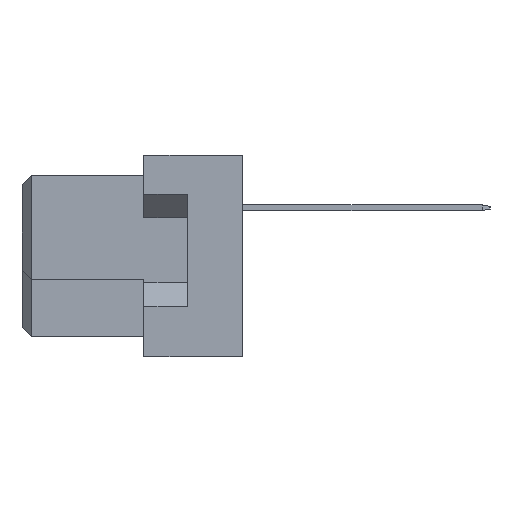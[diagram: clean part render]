
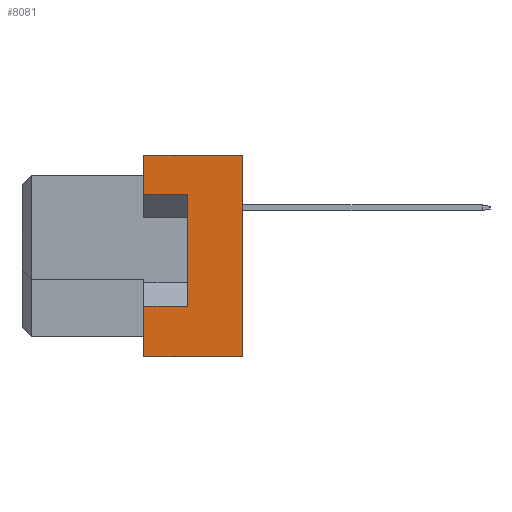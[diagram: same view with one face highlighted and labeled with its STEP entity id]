
A CAD part, left-side view. The second image highlights one B-rep face of the part: STEP entity #8081.
In plain terms, the highlighted planar face has unit normal (-1, 0, 0).
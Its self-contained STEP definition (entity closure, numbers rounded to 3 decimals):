
#211 = DIRECTION ( 'NONE',  ( 0., 0., 1. ) ) ;
#1290 = ORIENTED_EDGE ( 'NONE', *, *, #20643, .F. ) ;
#2016 = ORIENTED_EDGE ( 'NONE', *, *, #21092, .T. ) ;
#3316 = VERTEX_POINT ( 'NONE', #11749 ) ;
#4869 = CARTESIAN_POINT ( 'NONE',  ( -47.5, -11.6, 5.3 ) ) ;
#5547 = LINE ( 'NONE', #26498, #6067 ) ;
#5551 = VERTEX_POINT ( 'NONE', #25028 ) ;
#5770 = VERTEX_POINT ( 'NONE', #14816 ) ;
#5952 = DIRECTION ( 'NONE',  ( 0., 1., 0. ) ) ;
#6067 = VECTOR ( 'NONE', #8678, 1000. ) ;
#6468 = EDGE_CURVE ( 'NONE', #32099, #27374, #15330, .T. ) ;
#7495 = CARTESIAN_POINT ( 'NONE',  ( -47.5, -6.4, -2.65 ) ) ;
#7597 = DIRECTION ( 'NONE',  ( 0., 0., 1. ) ) ;
#7832 = VECTOR ( 'NONE', #8297, 1000. ) ;
#7844 = ORIENTED_EDGE ( 'NONE', *, *, #29473, .F. ) ;
#8081 = ADVANCED_FACE ( 'NONE', ( #37391 ), #34633, .T. ) ;
#8297 = DIRECTION ( 'NONE',  ( 0., 1., 0. ) ) ;
#8309 = VECTOR ( 'NONE', #35183, 1000. ) ;
#8678 = DIRECTION ( 'NONE',  ( 0., 0., 1. ) ) ;
#9259 = CARTESIAN_POINT ( 'NONE',  ( -47.5, -8.7, -2.65 ) ) ;
#11006 = VERTEX_POINT ( 'NONE', #27903 ) ;
#11712 = ORIENTED_EDGE ( 'NONE', *, *, #31493, .F. ) ;
#11749 = CARTESIAN_POINT ( 'NONE',  ( -47.5, -6.4, -5.3 ) ) ;
#12090 = VERTEX_POINT ( 'NONE', #22367 ) ;
#12371 = CARTESIAN_POINT ( 'NONE',  ( -47.5, -11.6, 5.3 ) ) ;
#12782 = VECTOR ( 'NONE', #36684, 1000. ) ;
#13508 = CARTESIAN_POINT ( 'NONE',  ( -47.5, -6.4, -5.3 ) ) ;
#14209 = CARTESIAN_POINT ( 'NONE',  ( -47.5, -11.6, -5.3 ) ) ;
#14816 = CARTESIAN_POINT ( 'NONE',  ( -47.5, -11.6, -5.3 ) ) ;
#14832 = LINE ( 'NONE', #23255, #8309 ) ;
#15099 = LINE ( 'NONE', #12371, #36594 ) ;
#15330 = LINE ( 'NONE', #27853, #12782 ) ;
#17097 = ORIENTED_EDGE ( 'NONE', *, *, #6468, .T. ) ;
#17341 = CARTESIAN_POINT ( 'NONE',  ( -47.5, -8.7, 3.25 ) ) ;
#17497 = LINE ( 'NONE', #9259, #27055 ) ;
#19231 = VECTOR ( 'NONE', #5952, 1000. ) ;
#20643 = EDGE_CURVE ( 'NONE', #3316, #27374, #22922, .T. ) ;
#21092 = EDGE_CURVE ( 'NONE', #12090, #30761, #14832, .T. ) ;
#22367 = CARTESIAN_POINT ( 'NONE',  ( -47.5, -11.6, 5.3 ) ) ;
#22519 = DIRECTION ( 'NONE',  ( -1., 0., 0. ) ) ;
#22922 = LINE ( 'NONE', #13508, #32128 ) ;
#23255 = CARTESIAN_POINT ( 'NONE',  ( -47.5, -11.6, 5.3 ) ) ;
#23553 = AXIS2_PLACEMENT_3D ( 'NONE', #4869, #22519, #7597 ) ;
#24830 = ORIENTED_EDGE ( 'NONE', *, *, #25033, .F. ) ;
#25028 = CARTESIAN_POINT ( 'NONE',  ( -47.5, -8.7, 3.25 ) ) ;
#25033 = EDGE_CURVE ( 'NONE', #11006, #30761, #5547, .T. ) ;
#25464 = DIRECTION ( 'NONE',  ( 0., 0., 1. ) ) ;
#26498 = CARTESIAN_POINT ( 'NONE',  ( -47.5, -6.4, -5.3 ) ) ;
#26584 = CARTESIAN_POINT ( 'NONE',  ( -47.5, -6.4, 5.3 ) ) ;
#27055 = VECTOR ( 'NONE', #29443, 1000. ) ;
#27374 = VERTEX_POINT ( 'NONE', #7495 ) ;
#27816 = CARTESIAN_POINT ( 'NONE',  ( -47.5, -8.7, -2.65 ) ) ;
#27853 = CARTESIAN_POINT ( 'NONE',  ( -47.5, -8.7, -2.65 ) ) ;
#27903 = CARTESIAN_POINT ( 'NONE',  ( -47.5, -6.4, 3.25 ) ) ;
#28815 = EDGE_CURVE ( 'NONE', #5770, #12090, #15099, .T. ) ;
#29443 = DIRECTION ( 'NONE',  ( 0., 0., 1. ) ) ;
#29473 = EDGE_CURVE ( 'NONE', #5770, #3316, #32223, .T. ) ;
#30761 = VERTEX_POINT ( 'NONE', #26584 ) ;
#31493 = EDGE_CURVE ( 'NONE', #5551, #11006, #32614, .T. ) ;
#31628 = ORIENTED_EDGE ( 'NONE', *, *, #28815, .T. ) ;
#32099 = VERTEX_POINT ( 'NONE', #27816 ) ;
#32128 = VECTOR ( 'NONE', #25464, 1000. ) ;
#32223 = LINE ( 'NONE', #14209, #7832 ) ;
#32614 = LINE ( 'NONE', #17341, #19231 ) ;
#34633 = PLANE ( 'NONE',  #23553 ) ;
#35183 = DIRECTION ( 'NONE',  ( 0., 1., 0. ) ) ;
#36216 = EDGE_LOOP ( 'NONE', ( #17097, #1290, #7844, #31628, #2016, #24830, #11712, #38512 ) ) ;
#36503 = EDGE_CURVE ( 'NONE', #32099, #5551, #17497, .T. ) ;
#36594 = VECTOR ( 'NONE', #211, 1000. ) ;
#36684 = DIRECTION ( 'NONE',  ( 0., 1., 0. ) ) ;
#37391 = FACE_OUTER_BOUND ( 'NONE', #36216, .T. ) ;
#38512 = ORIENTED_EDGE ( 'NONE', *, *, #36503, .F. ) ;
